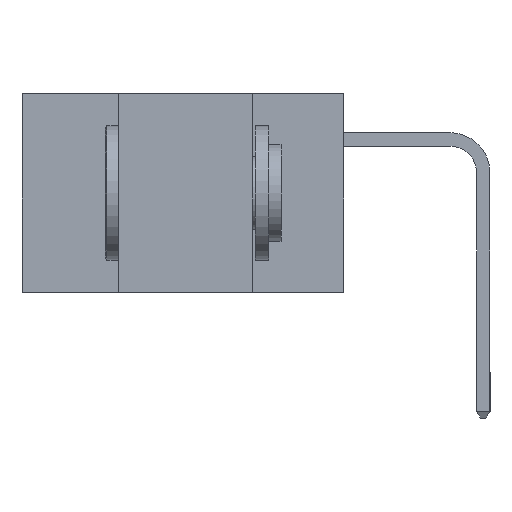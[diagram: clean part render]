
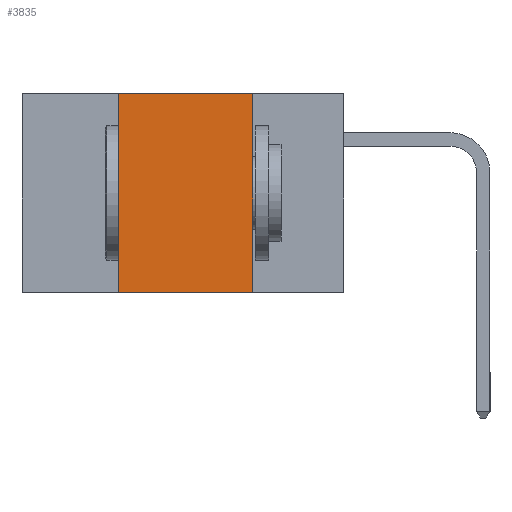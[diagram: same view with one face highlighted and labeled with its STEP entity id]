
A CAD part, left-side view. The second image highlights one B-rep face of the part: STEP entity #3835.
In plain terms, the highlighted planar face has unit normal (-1, 0, 0).
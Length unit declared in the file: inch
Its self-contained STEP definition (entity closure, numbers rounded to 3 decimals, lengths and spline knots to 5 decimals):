
#315 = EDGE_CURVE ( 'NONE', #2920, #7805, #6507, .T. ) ;
#394 = EDGE_LOOP ( 'NONE', ( #10670, #5963, #9110, #10636 ) ) ;
#622 = EDGE_CURVE ( 'NONE', #2920, #4166, #9728, .T. ) ;
#1045 = DIRECTION ( 'NONE',  ( 0., 0., 1. ) ) ;
#1650 = VERTEX_POINT ( 'NONE', #6012 ) ;
#1690 = VECTOR ( 'NONE', #6554, 39.37008 ) ;
#1971 = CARTESIAN_POINT ( 'NONE',  ( 0., 0.17, -0.37 ) ) ;
#2242 = CARTESIAN_POINT ( 'NONE',  ( 0., 0.42, -0.37 ) ) ;
#2920 = VERTEX_POINT ( 'NONE', #2242 ) ;
#3563 = CARTESIAN_POINT ( 'NONE',  ( 0., 0.42, -0.37 ) ) ;
#3835 = ADVANCED_FACE ( 'NONE', ( #9790 ), #4608, .F. ) ;
#3854 = VECTOR ( 'NONE', #1045, 39.37008 ) ;
#4110 = VECTOR ( 'NONE', #4876, 39.37008 ) ;
#4166 = VERTEX_POINT ( 'NONE', #6040 ) ;
#4608 = PLANE ( 'NONE',  #9678 ) ;
#4876 = DIRECTION ( 'NONE',  ( 0., -1., 0. ) ) ;
#5360 = EDGE_CURVE ( 'NONE', #1650, #7805, #10504, .T. ) ;
#5963 = ORIENTED_EDGE ( 'NONE', *, *, #7092, .F. ) ;
#6012 = CARTESIAN_POINT ( 'NONE',  ( 0., 0.17, 0. ) ) ;
#6040 = CARTESIAN_POINT ( 'NONE',  ( 0., 0.42, 0. ) ) ;
#6507 = LINE ( 'NONE', #9949, #1690 ) ;
#6554 = DIRECTION ( 'NONE',  ( 0., -1., 0. ) ) ;
#7092 = EDGE_CURVE ( 'NONE', #4166, #1650, #7511, .T. ) ;
#7245 = DIRECTION ( 'NONE',  ( 0., 0., -1. ) ) ;
#7409 = CARTESIAN_POINT ( 'NONE',  ( 0., 0.6, 0. ) ) ;
#7511 = LINE ( 'NONE', #9323, #4110 ) ;
#7805 = VERTEX_POINT ( 'NONE', #1971 ) ;
#8157 = DIRECTION ( 'NONE',  ( 1., 0., 0. ) ) ;
#9110 = ORIENTED_EDGE ( 'NONE', *, *, #622, .F. ) ;
#9323 = CARTESIAN_POINT ( 'NONE',  ( 0., 0.6, 0. ) ) ;
#9494 = DIRECTION ( 'NONE',  ( 0., 0., -1. ) ) ;
#9553 = CARTESIAN_POINT ( 'NONE',  ( 0., 0.17, -0.37 ) ) ;
#9678 = AXIS2_PLACEMENT_3D ( 'NONE', #7409, #8157, #7245 ) ;
#9728 = LINE ( 'NONE', #3563, #3854 ) ;
#9790 = FACE_OUTER_BOUND ( 'NONE', #394, .T. ) ;
#9949 = CARTESIAN_POINT ( 'NONE',  ( 0., 0.6, -0.37 ) ) ;
#10232 = VECTOR ( 'NONE', #9494, 39.37008 ) ;
#10504 = LINE ( 'NONE', #9553, #10232 ) ;
#10636 = ORIENTED_EDGE ( 'NONE', *, *, #315, .T. ) ;
#10670 = ORIENTED_EDGE ( 'NONE', *, *, #5360, .F. ) ;
